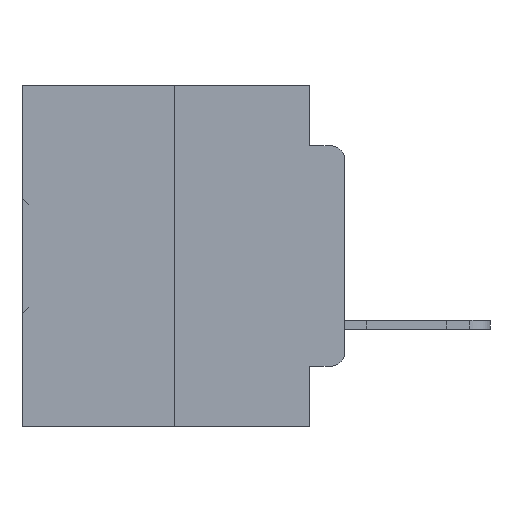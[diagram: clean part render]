
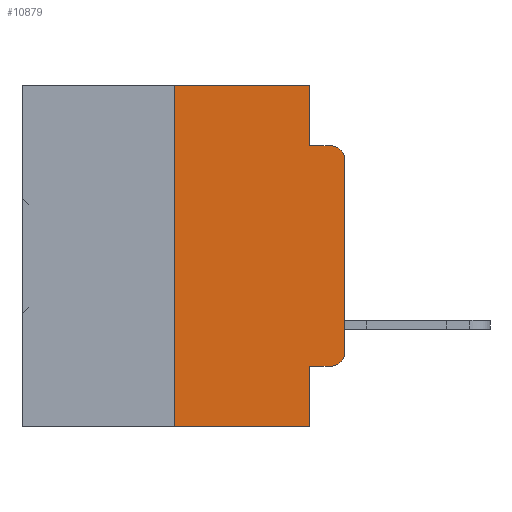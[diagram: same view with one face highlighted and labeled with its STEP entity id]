
A CAD part, left-side view. The second image highlights one B-rep face of the part: STEP entity #10879.
In plain terms, the highlighted planar face has unit normal (-1, 0, 0).
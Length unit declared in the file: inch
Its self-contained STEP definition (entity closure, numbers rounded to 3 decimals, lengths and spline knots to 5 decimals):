
#73 = CARTESIAN_POINT ( 'NONE',  ( 0., 0.02, -0.4115 ) ) ;
#470 = CARTESIAN_POINT ( 'NONE',  ( 0., 0.473, 0. ) ) ;
#547 = DIRECTION ( 'NONE',  ( 0., 0., 1. ) ) ;
#759 = ORIENTED_EDGE ( 'NONE', *, *, #22452, .F. ) ;
#1951 = EDGE_CURVE ( 'NONE', #28113, #5055, #21347, .T. ) ;
#2038 = LINE ( 'NONE', #10969, #15967 ) ;
#2041 = DIRECTION ( 'NONE',  ( 0., 0., 1. ) ) ;
#2294 = DIRECTION ( 'NONE',  ( 0., 0., -1. ) ) ;
#2391 = VERTEX_POINT ( 'NONE', #4972 ) ;
#3005 = VECTOR ( 'NONE', #25123, 39.37008 ) ;
#3216 = DIRECTION ( 'NONE',  ( 0., -1., 0. ) ) ;
#3434 = AXIS2_PLACEMENT_3D ( 'NONE', #34022, #16795, #36844 ) ;
#3683 = ORIENTED_EDGE ( 'NONE', *, *, #1951, .T. ) ;
#3990 = VECTOR ( 'NONE', #31546, 39.37008 ) ;
#4534 = PLANE ( 'NONE',  #5865 ) ;
#4972 = CARTESIAN_POINT ( 'NONE',  ( 0., 0.051, -0.0885 ) ) ;
#5055 = VERTEX_POINT ( 'NONE', #73 ) ;
#5144 = EDGE_CURVE ( 'NONE', #18666, #22917, #23406, .T. ) ;
#5774 = VECTOR ( 'NONE', #21663, 39.37008 ) ;
#5865 = AXIS2_PLACEMENT_3D ( 'NONE', #21982, #13432, #33622 ) ;
#7670 = VERTEX_POINT ( 'NONE', #31437 ) ;
#7903 = ORIENTED_EDGE ( 'NONE', *, *, #11317, .T. ) ;
#8262 = CARTESIAN_POINT ( 'NONE',  ( 0., 0., -0.3915 ) ) ;
#8833 = EDGE_CURVE ( 'NONE', #2391, #36734, #11105, .T. ) ;
#8928 = EDGE_LOOP ( 'NONE', ( #7903, #34581, #29660, #17999, #12043, #12953, #29218, #759, #3683, #28794 ) ) ;
#9498 = LINE ( 'NONE', #27569, #16319 ) ;
#9928 = VECTOR ( 'NONE', #547, 39.37008 ) ;
#10199 = VECTOR ( 'NONE', #3216, 39.37008 ) ;
#10879 = ADVANCED_FACE ( 'NONE', ( #30434 ), #4534, .F. ) ;
#10969 = CARTESIAN_POINT ( 'NONE',  ( 0., 0., 0. ) ) ;
#11105 = LINE ( 'NONE', #29244, #10199 ) ;
#11146 = VERTEX_POINT ( 'NONE', #34850 ) ;
#11317 = EDGE_CURVE ( 'NONE', #29929, #11146, #2038, .T. ) ;
#11456 = CIRCLE ( 'NONE', #22879, 0.02 ) ;
#11871 = LINE ( 'NONE', #16424, #3005 ) ;
#12043 = ORIENTED_EDGE ( 'NONE', *, *, #5144, .F. ) ;
#12118 = VERTEX_POINT ( 'NONE', #15387 ) ;
#12953 = ORIENTED_EDGE ( 'NONE', *, *, #24372, .F. ) ;
#13432 = DIRECTION ( 'NONE',  ( 1., 0., 0. ) ) ;
#15051 = CARTESIAN_POINT ( 'NONE',  ( 0., 0.02, -0.0885 ) ) ;
#15387 = CARTESIAN_POINT ( 'NONE',  ( 0., 0.051, -0.5 ) ) ;
#15692 = VECTOR ( 'NONE', #21240, 39.37008 ) ;
#15967 = VECTOR ( 'NONE', #2041, 39.37008 ) ;
#16084 = DIRECTION ( 'NONE',  ( 0., 0., -1. ) ) ;
#16319 = VECTOR ( 'NONE', #16084, 39.37008 ) ;
#16424 = CARTESIAN_POINT ( 'NONE',  ( 0., 0.051, 0. ) ) ;
#16795 = DIRECTION ( 'NONE',  ( -1., 0., 0. ) ) ;
#17999 = ORIENTED_EDGE ( 'NONE', *, *, #27516, .F. ) ;
#18666 = VERTEX_POINT ( 'NONE', #32145 ) ;
#18870 = CARTESIAN_POINT ( 'NONE',  ( 0., 0.051, -0.4115 ) ) ;
#19995 = DIRECTION ( 'NONE',  ( -1., 0., 0. ) ) ;
#21240 = DIRECTION ( 'NONE',  ( 0., -1., 0. ) ) ;
#21347 = LINE ( 'NONE', #22123, #5774 ) ;
#21663 = DIRECTION ( 'NONE',  ( 0., -1., 0. ) ) ;
#21982 = CARTESIAN_POINT ( 'NONE',  ( 0., 0.473, 0. ) ) ;
#22002 = EDGE_CURVE ( 'NONE', #7670, #12118, #34914, .T. ) ;
#22123 = CARTESIAN_POINT ( 'NONE',  ( 0., 0.051, -0.4115 ) ) ;
#22452 = EDGE_CURVE ( 'NONE', #28113, #12118, #11871, .T. ) ;
#22879 = AXIS2_PLACEMENT_3D ( 'NONE', #37111, #19995, #2294 ) ;
#22917 = VERTEX_POINT ( 'NONE', #25911 ) ;
#22918 = CARTESIAN_POINT ( 'NONE',  ( 0., 0.473, -0.5 ) ) ;
#23406 = LINE ( 'NONE', #470, #15692 ) ;
#24372 = EDGE_CURVE ( 'NONE', #7670, #18666, #32965, .T. ) ;
#25123 = DIRECTION ( 'NONE',  ( 0., 0., -1. ) ) ;
#25911 = CARTESIAN_POINT ( 'NONE',  ( 0., 0.051, 0. ) ) ;
#27516 = EDGE_CURVE ( 'NONE', #22917, #2391, #9498, .T. ) ;
#27569 = CARTESIAN_POINT ( 'NONE',  ( 0., 0.051, 0. ) ) ;
#28113 = VERTEX_POINT ( 'NONE', #18870 ) ;
#28794 = ORIENTED_EDGE ( 'NONE', *, *, #37754, .T. ) ;
#29023 = CIRCLE ( 'NONE', #3434, 0.02 ) ;
#29218 = ORIENTED_EDGE ( 'NONE', *, *, #22002, .T. ) ;
#29244 = CARTESIAN_POINT ( 'NONE',  ( 0., 0.051, -0.0885 ) ) ;
#29660 = ORIENTED_EDGE ( 'NONE', *, *, #8833, .F. ) ;
#29700 = CARTESIAN_POINT ( 'NONE',  ( 0., 0.25, 0. ) ) ;
#29929 = VERTEX_POINT ( 'NONE', #8262 ) ;
#30434 = FACE_OUTER_BOUND ( 'NONE', #8928, .T. ) ;
#31437 = CARTESIAN_POINT ( 'NONE',  ( 0., 0.25, -0.5 ) ) ;
#31546 = DIRECTION ( 'NONE',  ( 0., -1., 0. ) ) ;
#32145 = CARTESIAN_POINT ( 'NONE',  ( 0., 0.25, 0. ) ) ;
#32965 = LINE ( 'NONE', #29700, #9928 ) ;
#33622 = DIRECTION ( 'NONE',  ( 0., 0., -1. ) ) ;
#34022 = CARTESIAN_POINT ( 'NONE',  ( 0., 0.02, -0.3915 ) ) ;
#34581 = ORIENTED_EDGE ( 'NONE', *, *, #35222, .T. ) ;
#34850 = CARTESIAN_POINT ( 'NONE',  ( 0., 0., -0.1085 ) ) ;
#34914 = LINE ( 'NONE', #22918, #3990 ) ;
#35222 = EDGE_CURVE ( 'NONE', #11146, #36734, #11456, .T. ) ;
#36734 = VERTEX_POINT ( 'NONE', #15051 ) ;
#36844 = DIRECTION ( 'NONE',  ( 0., 0., -1. ) ) ;
#37111 = CARTESIAN_POINT ( 'NONE',  ( 0., 0.02, -0.1085 ) ) ;
#37754 = EDGE_CURVE ( 'NONE', #5055, #29929, #29023, .T. ) ;
